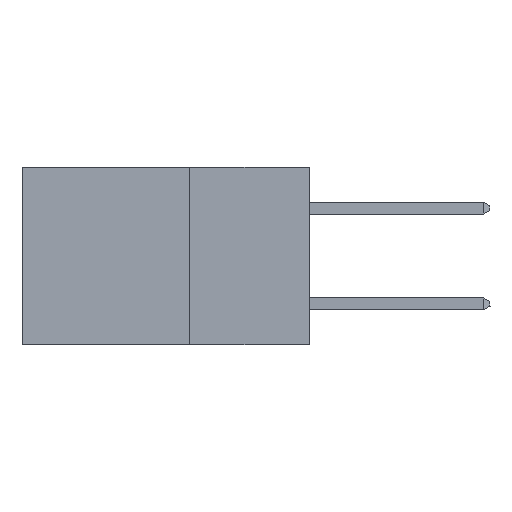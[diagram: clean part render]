
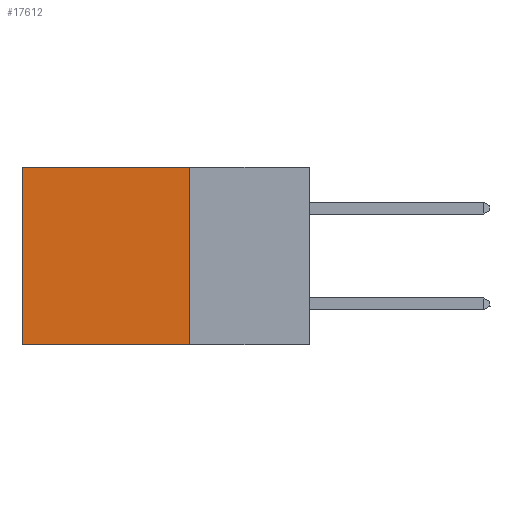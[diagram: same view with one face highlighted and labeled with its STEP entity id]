
A CAD part, left-side view. The second image highlights one B-rep face of the part: STEP entity #17612.
In plain terms, the highlighted planar face has unit normal (-1, 0, 0).
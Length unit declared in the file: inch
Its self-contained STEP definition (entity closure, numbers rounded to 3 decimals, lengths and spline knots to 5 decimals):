
#388 = CARTESIAN_POINT ( 'NONE',  ( 0.2875, 0.6, 0. ) ) ;
#1405 = DIRECTION ( 'NONE',  ( 0., 0., -1. ) ) ;
#1635 = CARTESIAN_POINT ( 'NONE',  ( 0.2875, 0.6, 0. ) ) ;
#1739 = CARTESIAN_POINT ( 'NONE',  ( 0.2875, 0.25, -0.37 ) ) ;
#1804 = CARTESIAN_POINT ( 'NONE',  ( 0.2875, 0.25, 0. ) ) ;
#2832 = AXIS2_PLACEMENT_3D ( 'NONE', #14581, #22680, #1405 ) ;
#4266 = DIRECTION ( 'NONE',  ( 0., 1., 0. ) ) ;
#5116 = VECTOR ( 'NONE', #4266, 39.37008 ) ;
#5197 = EDGE_CURVE ( 'NONE', #10799, #25601, #22729, .T. ) ;
#6369 = LINE ( 'NONE', #388, #33036 ) ;
#10799 = VERTEX_POINT ( 'NONE', #28836 ) ;
#11378 = CARTESIAN_POINT ( 'NONE',  ( 0.2875, 0.25, 0. ) ) ;
#11520 = EDGE_CURVE ( 'NONE', #10799, #21472, #24406, .T. ) ;
#13955 = VECTOR ( 'NONE', #16923, 39.37008 ) ;
#14402 = ORIENTED_EDGE ( 'NONE', *, *, #11520, .F. ) ;
#14581 = CARTESIAN_POINT ( 'NONE',  ( 0.2875, 0.25, 0. ) ) ;
#15855 = EDGE_CURVE ( 'NONE', #21472, #18752, #27636, .T. ) ;
#16663 = VECTOR ( 'NONE', #19135, 39.37008 ) ;
#16923 = DIRECTION ( 'NONE',  ( 0., 1., 0. ) ) ;
#17612 = ADVANCED_FACE ( 'NONE', ( #33046 ), #25486, .F. ) ;
#18752 = VERTEX_POINT ( 'NONE', #25803 ) ;
#19135 = DIRECTION ( 'NONE',  ( 0., 0., -1. ) ) ;
#19383 = DIRECTION ( 'NONE',  ( 0., 0., -1. ) ) ;
#21472 = VERTEX_POINT ( 'NONE', #1739 ) ;
#22487 = EDGE_LOOP ( 'NONE', ( #27066, #33864, #14402, #23994 ) ) ;
#22680 = DIRECTION ( 'NONE',  ( 1., 0., 0. ) ) ;
#22729 = LINE ( 'NONE', #1804, #5116 ) ;
#23994 = ORIENTED_EDGE ( 'NONE', *, *, #5197, .T. ) ;
#24406 = LINE ( 'NONE', #11378, #16663 ) ;
#25486 = PLANE ( 'NONE',  #2832 ) ;
#25601 = VERTEX_POINT ( 'NONE', #1635 ) ;
#25803 = CARTESIAN_POINT ( 'NONE',  ( 0.2875, 0.6, -0.37 ) ) ;
#26539 = EDGE_CURVE ( 'NONE', #25601, #18752, #6369, .T. ) ;
#27066 = ORIENTED_EDGE ( 'NONE', *, *, #26539, .T. ) ;
#27636 = LINE ( 'NONE', #27982, #13955 ) ;
#27982 = CARTESIAN_POINT ( 'NONE',  ( 0.2875, 0.25, -0.37 ) ) ;
#28836 = CARTESIAN_POINT ( 'NONE',  ( 0.2875, 0.25, 0. ) ) ;
#33036 = VECTOR ( 'NONE', #19383, 39.37008 ) ;
#33046 = FACE_OUTER_BOUND ( 'NONE', #22487, .T. ) ;
#33864 = ORIENTED_EDGE ( 'NONE', *, *, #15855, .F. ) ;
